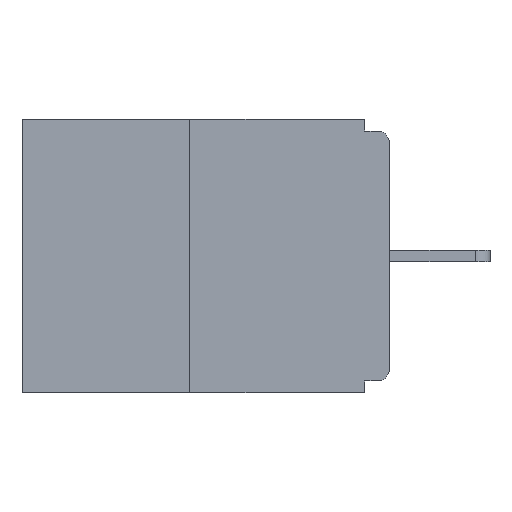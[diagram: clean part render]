
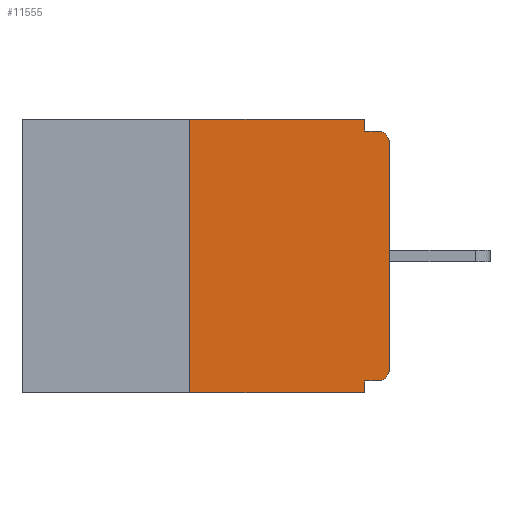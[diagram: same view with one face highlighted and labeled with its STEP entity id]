
A CAD part, left-side view. The second image highlights one B-rep face of the part: STEP entity #11555.
In plain terms, the highlighted planar face has unit normal (-1, 0, 0).
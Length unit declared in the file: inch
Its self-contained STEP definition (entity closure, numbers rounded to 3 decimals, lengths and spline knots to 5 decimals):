
#54 = CARTESIAN_POINT ( 'NONE',  ( 0., 0., -0.03 ) ) ;
#482 = ORIENTED_EDGE ( 'NONE', *, *, #11922, .F. ) ;
#649 = VERTEX_POINT ( 'NONE', #9616 ) ;
#662 = DIRECTION ( 'NONE',  ( 0., -1., 0. ) ) ;
#819 = ORIENTED_EDGE ( 'NONE', *, *, #18197, .T. ) ;
#988 = EDGE_CURVE ( 'NONE', #17889, #9302, #10081, .T. ) ;
#1137 = CARTESIAN_POINT ( 'NONE',  ( 0., 0.031, -0.015 ) ) ;
#1352 = CIRCLE ( 'NONE', #12071, 0.015 ) ;
#1385 = ORIENTED_EDGE ( 'NONE', *, *, #988, .F. ) ;
#1605 = CARTESIAN_POINT ( 'NONE',  ( 0., 0.25, 0. ) ) ;
#1863 = CARTESIAN_POINT ( 'NONE',  ( 0., 0.46, 0. ) ) ;
#2066 = VERTEX_POINT ( 'NONE', #10847 ) ;
#2248 = CARTESIAN_POINT ( 'NONE',  ( 0., 0.46, 0. ) ) ;
#2355 = CARTESIAN_POINT ( 'NONE',  ( 0., 0.46, -0.343 ) ) ;
#3314 = LINE ( 'NONE', #2355, #15276 ) ;
#3329 = DIRECTION ( 'NONE',  ( 0., 0., 1. ) ) ;
#3359 = VERTEX_POINT ( 'NONE', #21005 ) ;
#3484 = EDGE_CURVE ( 'NONE', #17117, #649, #1352, .T. ) ;
#3575 = EDGE_CURVE ( 'NONE', #16253, #3359, #12977, .T. ) ;
#3723 = ORIENTED_EDGE ( 'NONE', *, *, #3484, .T. ) ;
#5294 = VECTOR ( 'NONE', #10262, 39.37008 ) ;
#5378 = DIRECTION ( 'NONE',  ( 0., -1., 0. ) ) ;
#5590 = ORIENTED_EDGE ( 'NONE', *, *, #17383, .F. ) ;
#5802 = VECTOR ( 'NONE', #17321, 39.37008 ) ;
#6131 = CARTESIAN_POINT ( 'NONE',  ( 0., 0., 0. ) ) ;
#6262 = VERTEX_POINT ( 'NONE', #13378 ) ;
#7379 = DIRECTION ( 'NONE',  ( 1., 0., 0. ) ) ;
#7685 = ORIENTED_EDGE ( 'NONE', *, *, #13778, .F. ) ;
#7856 = VECTOR ( 'NONE', #9868, 39.37008 ) ;
#7865 = VECTOR ( 'NONE', #11654, 39.37008 ) ;
#8192 = CARTESIAN_POINT ( 'NONE',  ( 0., 0.031, -0.343 ) ) ;
#8426 = CARTESIAN_POINT ( 'NONE',  ( 0., 0.031, 0. ) ) ;
#8714 = CARTESIAN_POINT ( 'NONE',  ( 0., 0., -0.328 ) ) ;
#8852 = DIRECTION ( 'NONE',  ( 0., 0., -1. ) ) ;
#8888 = DIRECTION ( 'NONE',  ( -1., 0., 0. ) ) ;
#8954 = CARTESIAN_POINT ( 'NONE',  ( 0., 0.015, -0.03 ) ) ;
#9302 = VERTEX_POINT ( 'NONE', #1137 ) ;
#9502 = VECTOR ( 'NONE', #3329, 39.37008 ) ;
#9616 = CARTESIAN_POINT ( 'NONE',  ( 0., 0., -0.313 ) ) ;
#9647 = CARTESIAN_POINT ( 'NONE',  ( 0., 0.015, -0.328 ) ) ;
#9868 = DIRECTION ( 'NONE',  ( 0., 0., -1. ) ) ;
#9892 = CARTESIAN_POINT ( 'NONE',  ( 0., 0.031, -0.343 ) ) ;
#10003 = LINE ( 'NONE', #1605, #9502 ) ;
#10081 = LINE ( 'NONE', #19084, #11584 ) ;
#10234 = CARTESIAN_POINT ( 'NONE',  ( 0., 0., -0.015 ) ) ;
#10262 = DIRECTION ( 'NONE',  ( 0., 1., 0. ) ) ;
#10797 = EDGE_CURVE ( 'NONE', #6262, #17889, #15829, .T. ) ;
#10847 = CARTESIAN_POINT ( 'NONE',  ( 0., 0.25, -0.343 ) ) ;
#11555 = ADVANCED_FACE ( 'NONE', ( #15838 ), #16907, .F. ) ;
#11584 = VECTOR ( 'NONE', #20913, 39.37008 ) ;
#11654 = DIRECTION ( 'NONE',  ( 0., -1., 0. ) ) ;
#11922 = EDGE_CURVE ( 'NONE', #16960, #17845, #16320, .T. ) ;
#12036 = CARTESIAN_POINT ( 'NONE',  ( 0., 0.015, -0.313 ) ) ;
#12071 = AXIS2_PLACEMENT_3D ( 'NONE', #12036, #12329, #12316 ) ;
#12316 = DIRECTION ( 'NONE',  ( 0., 0., -1. ) ) ;
#12329 = DIRECTION ( 'NONE',  ( -1., 0., 0. ) ) ;
#12867 = EDGE_CURVE ( 'NONE', #2066, #17845, #3314, .T. ) ;
#12977 = CIRCLE ( 'NONE', #19477, 0.015 ) ;
#13099 = AXIS2_PLACEMENT_3D ( 'NONE', #2248, #7379, #18470 ) ;
#13378 = CARTESIAN_POINT ( 'NONE',  ( 0., 0.25, 0. ) ) ;
#13509 = EDGE_LOOP ( 'NONE', ( #17854, #7685, #18597, #482, #5590, #3723, #819, #16967, #15715, #1385 ) ) ;
#13778 = EDGE_CURVE ( 'NONE', #2066, #6262, #10003, .T. ) ;
#15100 = VECTOR ( 'NONE', #5378, 39.37008 ) ;
#15276 = VECTOR ( 'NONE', #662, 39.37008 ) ;
#15615 = CARTESIAN_POINT ( 'NONE',  ( 0., 0.031, -0.328 ) ) ;
#15715 = ORIENTED_EDGE ( 'NONE', *, *, #17945, .F. ) ;
#15829 = LINE ( 'NONE', #1863, #7865 ) ;
#15838 = FACE_OUTER_BOUND ( 'NONE', #13509, .T. ) ;
#16253 = VERTEX_POINT ( 'NONE', #54 ) ;
#16320 = LINE ( 'NONE', #8192, #7856 ) ;
#16907 = PLANE ( 'NONE',  #13099 ) ;
#16960 = VERTEX_POINT ( 'NONE', #15615 ) ;
#16967 = ORIENTED_EDGE ( 'NONE', *, *, #3575, .T. ) ;
#17117 = VERTEX_POINT ( 'NONE', #9647 ) ;
#17321 = DIRECTION ( 'NONE',  ( 0., 0., 1. ) ) ;
#17383 = EDGE_CURVE ( 'NONE', #17117, #16960, #18082, .T. ) ;
#17845 = VERTEX_POINT ( 'NONE', #9892 ) ;
#17854 = ORIENTED_EDGE ( 'NONE', *, *, #10797, .F. ) ;
#17889 = VERTEX_POINT ( 'NONE', #8426 ) ;
#17945 = EDGE_CURVE ( 'NONE', #9302, #3359, #19296, .T. ) ;
#18049 = LINE ( 'NONE', #6131, #5802 ) ;
#18082 = LINE ( 'NONE', #8714, #5294 ) ;
#18197 = EDGE_CURVE ( 'NONE', #649, #16253, #18049, .T. ) ;
#18470 = DIRECTION ( 'NONE',  ( 0., 0., -1. ) ) ;
#18597 = ORIENTED_EDGE ( 'NONE', *, *, #12867, .T. ) ;
#19084 = CARTESIAN_POINT ( 'NONE',  ( 0., 0.031, 0. ) ) ;
#19296 = LINE ( 'NONE', #10234, #15100 ) ;
#19477 = AXIS2_PLACEMENT_3D ( 'NONE', #8954, #8888, #8852 ) ;
#20913 = DIRECTION ( 'NONE',  ( 0., 0., -1. ) ) ;
#21005 = CARTESIAN_POINT ( 'NONE',  ( 0., 0.015, -0.015 ) ) ;
